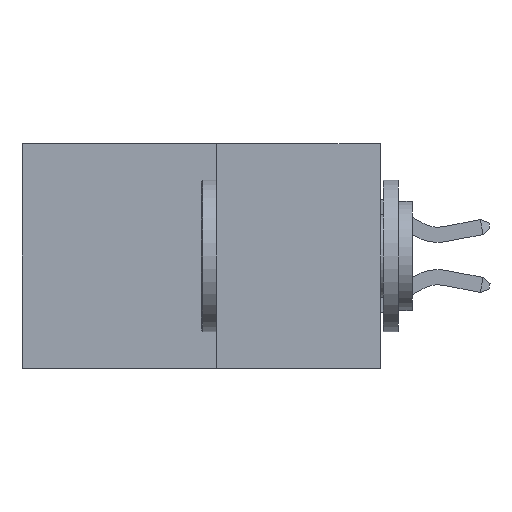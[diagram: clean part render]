
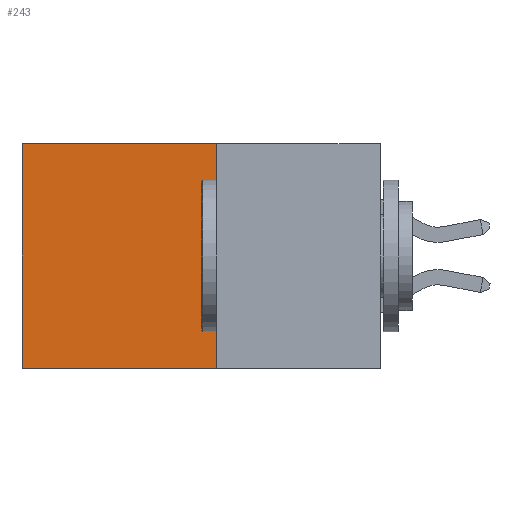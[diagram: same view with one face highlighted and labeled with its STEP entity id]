
A CAD part, left-side view. The second image highlights one B-rep face of the part: STEP entity #243.
In plain terms, the highlighted planar face has unit normal (-1, 0, 0).
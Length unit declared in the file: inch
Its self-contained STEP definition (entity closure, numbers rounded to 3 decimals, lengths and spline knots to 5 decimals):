
#113 = ORIENTED_EDGE ( 'NONE', *, *, #1244, .T. ) ;
#243 = ADVANCED_FACE ( 'NONE', ( #5434 ), #8980, .F. ) ;
#556 = CARTESIAN_POINT ( 'NONE',  ( 0.277, 0.27, 0. ) ) ;
#1244 = EDGE_CURVE ( 'NONE', #5512, #9206, #2492, .T. ) ;
#1269 = EDGE_CURVE ( 'NONE', #9206, #7883, #4218, .T. ) ;
#1891 = CARTESIAN_POINT ( 'NONE',  ( 0.277, 0.59, -0.37 ) ) ;
#2219 = VECTOR ( 'NONE', #11073, 39.37008 ) ;
#2434 = ORIENTED_EDGE ( 'NONE', *, *, #9520, .F. ) ;
#2492 = LINE ( 'NONE', #556, #2219 ) ;
#3140 = LINE ( 'NONE', #9750, #9412 ) ;
#3225 = CARTESIAN_POINT ( 'NONE',  ( 0.277, 0.27, -0.37 ) ) ;
#3651 = DIRECTION ( 'NONE',  ( 0., 0., -1. ) ) ;
#3832 = DIRECTION ( 'NONE',  ( 0., 1., 0. ) ) ;
#3908 = AXIS2_PLACEMENT_3D ( 'NONE', #9036, #7932, #9124 ) ;
#4218 = LINE ( 'NONE', #1891, #8497 ) ;
#4698 = ORIENTED_EDGE ( 'NONE', *, *, #8926, .F. ) ;
#5434 = FACE_OUTER_BOUND ( 'NONE', #7183, .T. ) ;
#5512 = VERTEX_POINT ( 'NONE', #8203 ) ;
#6911 = CARTESIAN_POINT ( 'NONE',  ( 0.277, 0.59, 0. ) ) ;
#7183 = EDGE_LOOP ( 'NONE', ( #11064, #2434, #4698, #113 ) ) ;
#7883 = VERTEX_POINT ( 'NONE', #10690 ) ;
#7932 = DIRECTION ( 'NONE',  ( 1., 0., 0. ) ) ;
#8203 = CARTESIAN_POINT ( 'NONE',  ( 0.277, 0.27, 0. ) ) ;
#8497 = VECTOR ( 'NONE', #3651, 39.37008 ) ;
#8926 = EDGE_CURVE ( 'NONE', #5512, #10151, #9552, .T. ) ;
#8980 = PLANE ( 'NONE',  #3908 ) ;
#9001 = VECTOR ( 'NONE', #10003, 39.37008 ) ;
#9036 = CARTESIAN_POINT ( 'NONE',  ( 0.277, 0.27, -0.37 ) ) ;
#9124 = DIRECTION ( 'NONE',  ( 0., 0., -1. ) ) ;
#9206 = VERTEX_POINT ( 'NONE', #6911 ) ;
#9412 = VECTOR ( 'NONE', #3832, 39.37008 ) ;
#9520 = EDGE_CURVE ( 'NONE', #10151, #7883, #3140, .T. ) ;
#9552 = LINE ( 'NONE', #3225, #9001 ) ;
#9750 = CARTESIAN_POINT ( 'NONE',  ( 0.277, 0.27, -0.37 ) ) ;
#10003 = DIRECTION ( 'NONE',  ( 0., 0., -1. ) ) ;
#10151 = VERTEX_POINT ( 'NONE', #10988 ) ;
#10690 = CARTESIAN_POINT ( 'NONE',  ( 0.277, 0.59, -0.37 ) ) ;
#10988 = CARTESIAN_POINT ( 'NONE',  ( 0.277, 0.27, -0.37 ) ) ;
#11064 = ORIENTED_EDGE ( 'NONE', *, *, #1269, .T. ) ;
#11073 = DIRECTION ( 'NONE',  ( 0., 1., 0. ) ) ;
